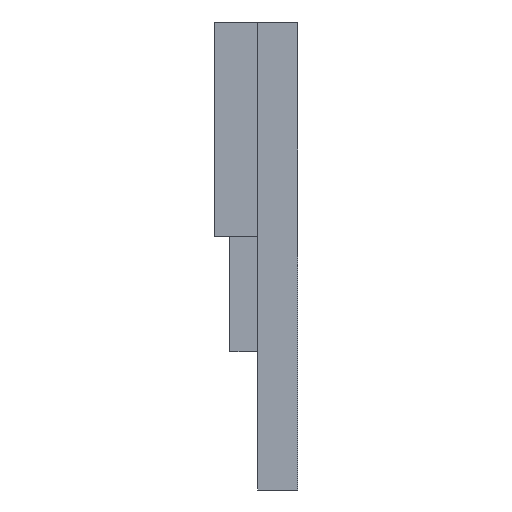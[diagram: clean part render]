
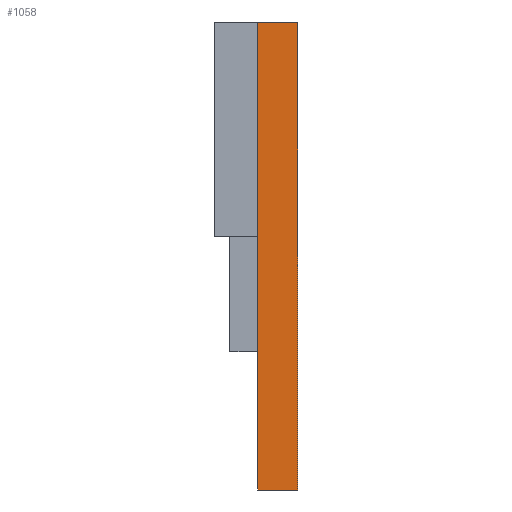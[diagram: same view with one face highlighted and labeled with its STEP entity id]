
A CAD part, left-side view. The second image highlights one B-rep face of the part: STEP entity #1058.
In plain terms, the highlighted planar face has unit normal (-1, 0, 0).
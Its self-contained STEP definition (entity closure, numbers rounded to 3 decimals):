
#7 = EDGE_CURVE ( 'NONE', #606, #871, #1308, .T. ) ;
#24 = LINE ( 'NONE', #929, #1462 ) ;
#117 = VERTEX_POINT ( 'NONE', #1140 ) ;
#384 = DIRECTION ( 'NONE',  ( 1., 0., 0. ) ) ;
#447 = CARTESIAN_POINT ( 'NONE',  ( -93.25, 0., 36.5 ) ) ;
#452 = VECTOR ( 'NONE', #731, 1000. ) ;
#484 = DIRECTION ( 'NONE',  ( 0., -1., 0. ) ) ;
#525 = EDGE_CURVE ( 'NONE', #606, #117, #24, .T. ) ;
#582 = VERTEX_POINT ( 'NONE', #794 ) ;
#606 = VERTEX_POINT ( 'NONE', #920 ) ;
#645 = EDGE_LOOP ( 'NONE', ( #1367, #1217, #1111, #1650 ) ) ;
#723 = FACE_OUTER_BOUND ( 'NONE', #645, .T. ) ;
#731 = DIRECTION ( 'NONE',  ( 0., -1., 0. ) ) ;
#739 = DIRECTION ( 'NONE',  ( 0., 0., 1. ) ) ;
#781 = VECTOR ( 'NONE', #484, 1000. ) ;
#789 = DIRECTION ( 'NONE',  ( 0., 0., -1. ) ) ;
#794 = CARTESIAN_POINT ( 'NONE',  ( -93.25, 0., 36.5 ) ) ;
#871 = VERTEX_POINT ( 'NONE', #1282 ) ;
#920 = CARTESIAN_POINT ( 'NONE',  ( -93.25, 6.3, -36.5 ) ) ;
#929 = CARTESIAN_POINT ( 'NONE',  ( -93.25, 6.3, 36.5 ) ) ;
#1035 = CARTESIAN_POINT ( 'NONE',  ( -93.25, 6.3, 36.5 ) ) ;
#1058 = ADVANCED_FACE ( 'NONE', ( #723 ), #1232, .F. ) ;
#1065 = LINE ( 'NONE', #447, #1638 ) ;
#1111 = ORIENTED_EDGE ( 'NONE', *, *, #525, .F. ) ;
#1140 = CARTESIAN_POINT ( 'NONE',  ( -93.25, 6.3, 36.5 ) ) ;
#1193 = AXIS2_PLACEMENT_3D ( 'NONE', #1629, #384, #789 ) ;
#1217 = ORIENTED_EDGE ( 'NONE', *, *, #1246, .F. ) ;
#1232 = PLANE ( 'NONE',  #1193 ) ;
#1246 = EDGE_CURVE ( 'NONE', #117, #582, #1470, .T. ) ;
#1282 = CARTESIAN_POINT ( 'NONE',  ( -93.25, 0., -36.5 ) ) ;
#1308 = LINE ( 'NONE', #1579, #452 ) ;
#1367 = ORIENTED_EDGE ( 'NONE', *, *, #1551, .T. ) ;
#1462 = VECTOR ( 'NONE', #1785, 1000. ) ;
#1470 = LINE ( 'NONE', #1035, #781 ) ;
#1551 = EDGE_CURVE ( 'NONE', #871, #582, #1065, .T. ) ;
#1579 = CARTESIAN_POINT ( 'NONE',  ( -93.25, 6.3, -36.5 ) ) ;
#1629 = CARTESIAN_POINT ( 'NONE',  ( -93.25, 6.3, 36.5 ) ) ;
#1638 = VECTOR ( 'NONE', #739, 1000. ) ;
#1650 = ORIENTED_EDGE ( 'NONE', *, *, #7, .T. ) ;
#1785 = DIRECTION ( 'NONE',  ( 0., 0., 1. ) ) ;
